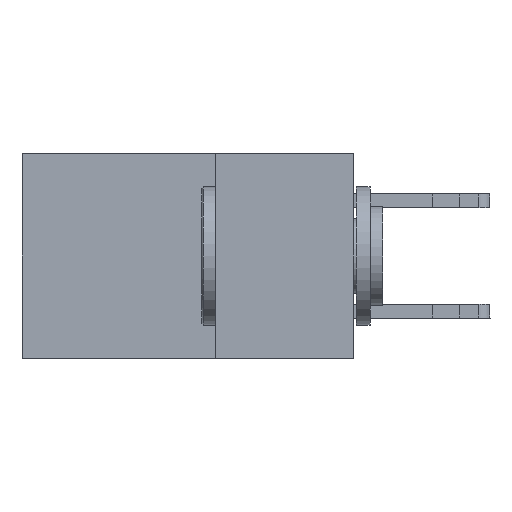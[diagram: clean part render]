
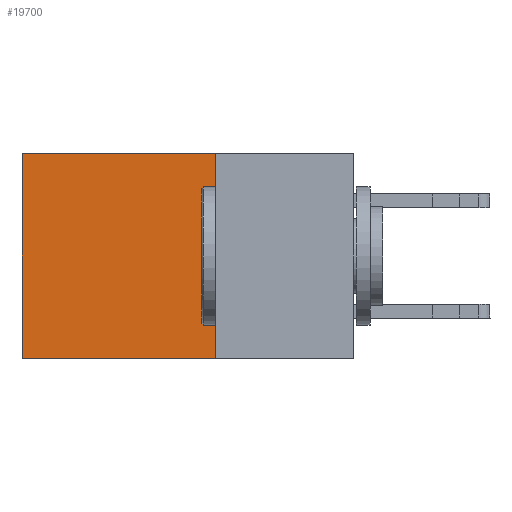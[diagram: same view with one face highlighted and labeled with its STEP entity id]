
A CAD part, left-side view. The second image highlights one B-rep face of the part: STEP entity #19700.
In plain terms, the highlighted planar face has unit normal (-1, 0, 0).
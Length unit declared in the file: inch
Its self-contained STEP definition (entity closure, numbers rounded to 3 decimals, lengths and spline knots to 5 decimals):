
#307 = LINE ( 'NONE', #12957, #9235 ) ;
#2254 = VECTOR ( 'NONE', #7022, 39.37008 ) ;
#2517 = CARTESIAN_POINT ( 'NONE',  ( 0.2875, 0.25, 0. ) ) ;
#3315 = LINE ( 'NONE', #10763, #15801 ) ;
#3989 = VECTOR ( 'NONE', #17610, 39.37008 ) ;
#4253 = DIRECTION ( 'NONE',  ( 1., 0., 0. ) ) ;
#4518 = LINE ( 'NONE', #20767, #3989 ) ;
#4706 = EDGE_CURVE ( 'NONE', #17175, #8780, #4518, .T. ) ;
#4735 = CARTESIAN_POINT ( 'NONE',  ( 0.2875, 0.25, -0.37 ) ) ;
#4817 = DIRECTION ( 'NONE',  ( 0., 1., 0. ) ) ;
#5184 = ORIENTED_EDGE ( 'NONE', *, *, #16535, .T. ) ;
#5442 = ORIENTED_EDGE ( 'NONE', *, *, #4706, .F. ) ;
#5887 = CARTESIAN_POINT ( 'NONE',  ( 0.2875, 0.6, -0.37 ) ) ;
#6130 = CARTESIAN_POINT ( 'NONE',  ( 0.2875, 0.6, 0. ) ) ;
#6917 = CARTESIAN_POINT ( 'NONE',  ( 0.2875, 0.25, 0. ) ) ;
#6975 = ORIENTED_EDGE ( 'NONE', *, *, #14609, .T. ) ;
#7022 = DIRECTION ( 'NONE',  ( 0., 0., -1. ) ) ;
#7255 = LINE ( 'NONE', #19874, #2254 ) ;
#7316 = AXIS2_PLACEMENT_3D ( 'NONE', #2517, #4253, #15605 ) ;
#8389 = FACE_OUTER_BOUND ( 'NONE', #11593, .T. ) ;
#8780 = VERTEX_POINT ( 'NONE', #4735 ) ;
#9235 = VECTOR ( 'NONE', #4817, 39.37008 ) ;
#9388 = ORIENTED_EDGE ( 'NONE', *, *, #17387, .F. ) ;
#10044 = VERTEX_POINT ( 'NONE', #6130 ) ;
#10763 = CARTESIAN_POINT ( 'NONE',  ( 0.2875, 0.25, -0.37 ) ) ;
#11593 = EDGE_LOOP ( 'NONE', ( #5184, #9388, #5442, #6975 ) ) ;
#12364 = DIRECTION ( 'NONE',  ( 0., 1., 0. ) ) ;
#12370 = PLANE ( 'NONE',  #7316 ) ;
#12957 = CARTESIAN_POINT ( 'NONE',  ( 0.2875, 0.25, 0. ) ) ;
#14609 = EDGE_CURVE ( 'NONE', #17175, #10044, #307, .T. ) ;
#15605 = DIRECTION ( 'NONE',  ( 0., 0., -1. ) ) ;
#15801 = VECTOR ( 'NONE', #12364, 39.37008 ) ;
#16535 = EDGE_CURVE ( 'NONE', #10044, #20920, #7255, .T. ) ;
#17175 = VERTEX_POINT ( 'NONE', #6917 ) ;
#17387 = EDGE_CURVE ( 'NONE', #8780, #20920, #3315, .T. ) ;
#17610 = DIRECTION ( 'NONE',  ( 0., 0., -1. ) ) ;
#19700 = ADVANCED_FACE ( 'NONE', ( #8389 ), #12370, .F. ) ;
#19874 = CARTESIAN_POINT ( 'NONE',  ( 0.2875, 0.6, 0. ) ) ;
#20767 = CARTESIAN_POINT ( 'NONE',  ( 0.2875, 0.25, 0. ) ) ;
#20920 = VERTEX_POINT ( 'NONE', #5887 ) ;
